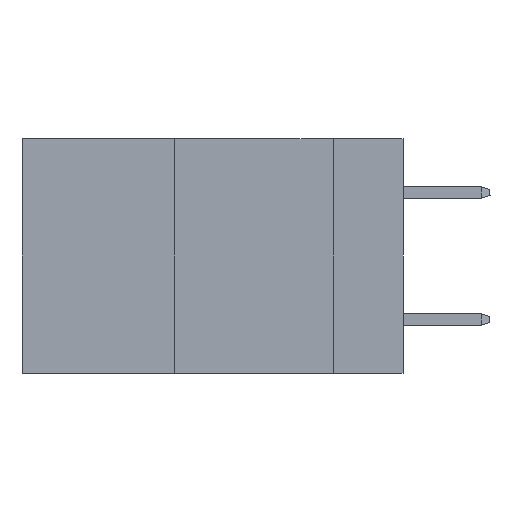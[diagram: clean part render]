
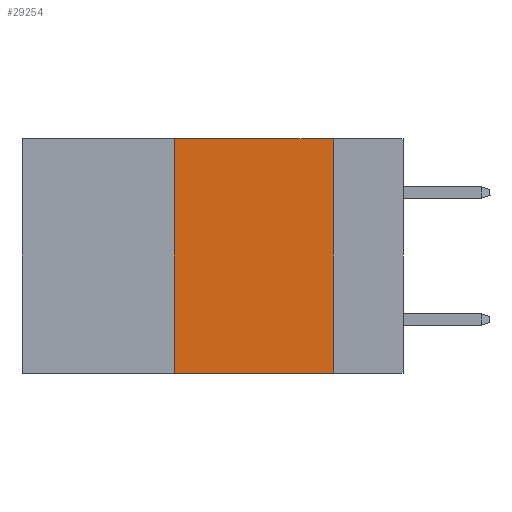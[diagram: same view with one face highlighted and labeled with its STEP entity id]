
A CAD part, left-side view. The second image highlights one B-rep face of the part: STEP entity #29254.
In plain terms, the highlighted planar face has unit normal (-1, 0, 0).
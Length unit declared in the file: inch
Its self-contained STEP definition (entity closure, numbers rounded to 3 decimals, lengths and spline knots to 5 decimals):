
#502 = ORIENTED_EDGE ( 'NONE', *, *, #18978, .F. ) ;
#667 = CARTESIAN_POINT ( 'NONE',  ( 0., 0.11, 0. ) ) ;
#1021 = VERTEX_POINT ( 'NONE', #31846 ) ;
#3681 = LINE ( 'NONE', #11725, #8763 ) ;
#4385 = LINE ( 'NONE', #31106, #14873 ) ;
#6215 = DIRECTION ( 'NONE',  ( 0., 0., -1. ) ) ;
#6869 = VERTEX_POINT ( 'NONE', #34308 ) ;
#7174 = DIRECTION ( 'NONE',  ( 0., -1., 0. ) ) ;
#8473 = DIRECTION ( 'NONE',  ( 0., 0., 1. ) ) ;
#8753 = DIRECTION ( 'NONE',  ( 0., -1., 0. ) ) ;
#8763 = VECTOR ( 'NONE', #8753, 39.37008 ) ;
#11725 = CARTESIAN_POINT ( 'NONE',  ( 0., 0.6, 0. ) ) ;
#11973 = PLANE ( 'NONE',  #13707 ) ;
#13707 = AXIS2_PLACEMENT_3D ( 'NONE', #30147, #32955, #6215 ) ;
#14775 = EDGE_CURVE ( 'NONE', #1021, #6869, #4385, .T. ) ;
#14873 = VECTOR ( 'NONE', #7174, 39.37008 ) ;
#18067 = VERTEX_POINT ( 'NONE', #19541 ) ;
#18978 = EDGE_CURVE ( 'NONE', #1021, #18067, #24549, .T. ) ;
#19541 = CARTESIAN_POINT ( 'NONE',  ( 0., 0.36, 0. ) ) ;
#19584 = CARTESIAN_POINT ( 'NONE',  ( 0., 0.36, 0. ) ) ;
#20936 = VECTOR ( 'NONE', #8473, 39.37008 ) ;
#24549 = LINE ( 'NONE', #19584, #20936 ) ;
#25476 = ORIENTED_EDGE ( 'NONE', *, *, #33107, .F. ) ;
#27374 = LINE ( 'NONE', #667, #28929 ) ;
#28802 = ORIENTED_EDGE ( 'NONE', *, *, #34351, .F. ) ;
#28929 = VECTOR ( 'NONE', #32297, 39.37008 ) ;
#29254 = ADVANCED_FACE ( 'NONE', ( #33464 ), #11973, .F. ) ;
#30136 = VERTEX_POINT ( 'NONE', #31080 ) ;
#30147 = CARTESIAN_POINT ( 'NONE',  ( 0., 0.6, 0. ) ) ;
#30418 = ORIENTED_EDGE ( 'NONE', *, *, #14775, .T. ) ;
#31080 = CARTESIAN_POINT ( 'NONE',  ( 0., 0.11, 0. ) ) ;
#31106 = CARTESIAN_POINT ( 'NONE',  ( 0., 0.6, -0.37 ) ) ;
#31846 = CARTESIAN_POINT ( 'NONE',  ( 0., 0.36, -0.37 ) ) ;
#32297 = DIRECTION ( 'NONE',  ( 0., 0., -1. ) ) ;
#32955 = DIRECTION ( 'NONE',  ( 1., 0., 0. ) ) ;
#33107 = EDGE_CURVE ( 'NONE', #18067, #30136, #3681, .T. ) ;
#33464 = FACE_OUTER_BOUND ( 'NONE', #33631, .T. ) ;
#33631 = EDGE_LOOP ( 'NONE', ( #28802, #25476, #502, #30418 ) ) ;
#34308 = CARTESIAN_POINT ( 'NONE',  ( 0., 0.11, -0.37 ) ) ;
#34351 = EDGE_CURVE ( 'NONE', #30136, #6869, #27374, .T. ) ;
